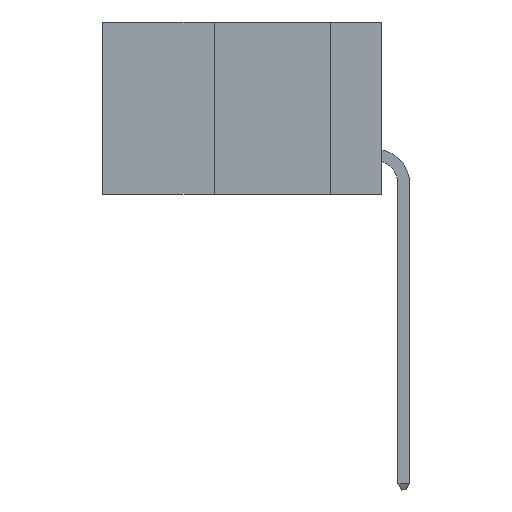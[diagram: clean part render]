
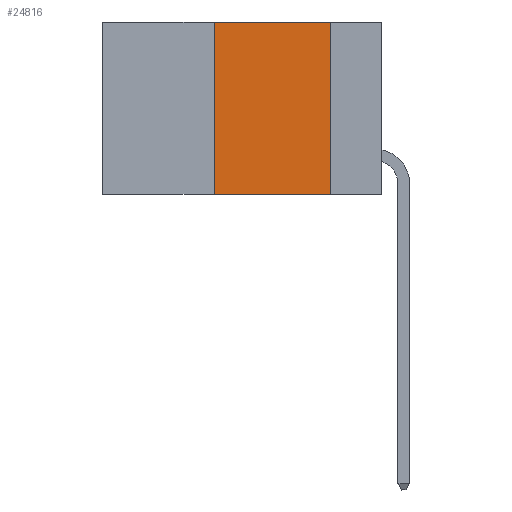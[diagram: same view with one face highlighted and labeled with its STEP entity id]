
A CAD part, left-side view. The second image highlights one B-rep face of the part: STEP entity #24816.
In plain terms, the highlighted planar face has unit normal (-1, 0, 0).
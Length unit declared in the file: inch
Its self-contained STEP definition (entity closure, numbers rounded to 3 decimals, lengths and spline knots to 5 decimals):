
#276 = CARTESIAN_POINT ( 'NONE',  ( 0., 0.36, 0. ) ) ;
#768 = DIRECTION ( 'NONE',  ( 1., 0., 0. ) ) ;
#1150 = VECTOR ( 'NONE', #17071, 39.37008 ) ;
#1805 = ORIENTED_EDGE ( 'NONE', *, *, #13556, .T. ) ;
#2602 = AXIS2_PLACEMENT_3D ( 'NONE', #25799, #768, #15411 ) ;
#2909 = CARTESIAN_POINT ( 'NONE',  ( 0., 0.36, 0. ) ) ;
#3892 = ORIENTED_EDGE ( 'NONE', *, *, #19227, .F. ) ;
#3966 = DIRECTION ( 'NONE',  ( 0., 0., 1. ) ) ;
#4689 = DIRECTION ( 'NONE',  ( 0., -1., 0. ) ) ;
#5001 = PLANE ( 'NONE',  #2602 ) ;
#5238 = EDGE_LOOP ( 'NONE', ( #7328, #22195, #3892, #1805 ) ) ;
#5345 = CARTESIAN_POINT ( 'NONE',  ( 0., 0.11, 0. ) ) ;
#6029 = VERTEX_POINT ( 'NONE', #17811 ) ;
#6638 = CARTESIAN_POINT ( 'NONE',  ( 0., 0.6, -0.37 ) ) ;
#7328 = ORIENTED_EDGE ( 'NONE', *, *, #10173, .F. ) ;
#7678 = LINE ( 'NONE', #10854, #22909 ) ;
#8721 = CARTESIAN_POINT ( 'NONE',  ( 0., 0.11, -0.37 ) ) ;
#10037 = VERTEX_POINT ( 'NONE', #8721 ) ;
#10173 = EDGE_CURVE ( 'NONE', #6029, #10037, #22881, .T. ) ;
#10854 = CARTESIAN_POINT ( 'NONE',  ( 0., 0.6, 0. ) ) ;
#12253 = EDGE_CURVE ( 'NONE', #25816, #6029, #7678, .T. ) ;
#13460 = FACE_OUTER_BOUND ( 'NONE', #5238, .T. ) ;
#13556 = EDGE_CURVE ( 'NONE', #26273, #10037, #22478, .T. ) ;
#13892 = CARTESIAN_POINT ( 'NONE',  ( 0., 0.36, -0.37 ) ) ;
#15411 = DIRECTION ( 'NONE',  ( 0., 0., -1. ) ) ;
#17071 = DIRECTION ( 'NONE',  ( 0., -1., 0. ) ) ;
#17811 = CARTESIAN_POINT ( 'NONE',  ( 0., 0.11, 0. ) ) ;
#19227 = EDGE_CURVE ( 'NONE', #26273, #25816, #25930, .T. ) ;
#19843 = DIRECTION ( 'NONE',  ( 0., 0., -1. ) ) ;
#21075 = VECTOR ( 'NONE', #3966, 39.37008 ) ;
#22195 = ORIENTED_EDGE ( 'NONE', *, *, #12253, .F. ) ;
#22478 = LINE ( 'NONE', #6638, #1150 ) ;
#22881 = LINE ( 'NONE', #5345, #24169 ) ;
#22909 = VECTOR ( 'NONE', #4689, 39.37008 ) ;
#24169 = VECTOR ( 'NONE', #19843, 39.37008 ) ;
#24816 = ADVANCED_FACE ( 'NONE', ( #13460 ), #5001, .F. ) ;
#25799 = CARTESIAN_POINT ( 'NONE',  ( 0., 0.6, 0. ) ) ;
#25816 = VERTEX_POINT ( 'NONE', #2909 ) ;
#25930 = LINE ( 'NONE', #276, #21075 ) ;
#26273 = VERTEX_POINT ( 'NONE', #13892 ) ;
